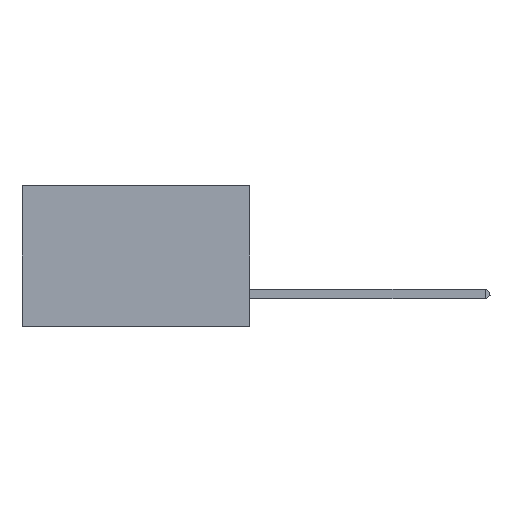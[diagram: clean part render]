
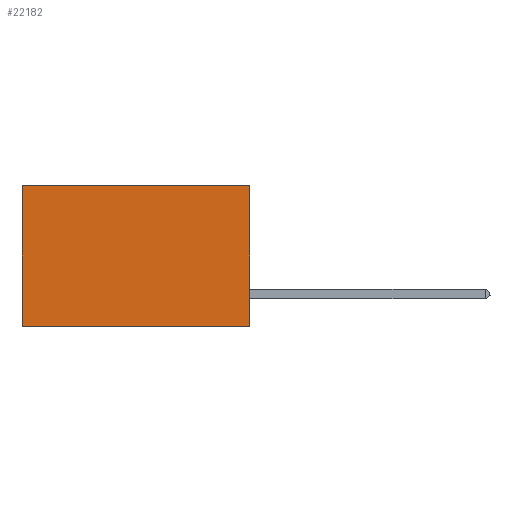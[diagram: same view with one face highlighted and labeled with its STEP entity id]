
A CAD part, left-side view. The second image highlights one B-rep face of the part: STEP entity #22182.
In plain terms, the highlighted planar face has unit normal (-1, 0, 0).
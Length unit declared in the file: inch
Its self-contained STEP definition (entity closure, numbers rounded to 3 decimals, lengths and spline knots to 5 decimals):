
#1381 = CARTESIAN_POINT ( 'NONE',  ( 0.2875, 0., 0. ) ) ;
#2530 = EDGE_CURVE ( 'NONE', #5584, #11967, #15903, .T. ) ;
#3696 = CARTESIAN_POINT ( 'NONE',  ( 0.2875, 0., 0. ) ) ;
#5584 = VERTEX_POINT ( 'NONE', #42469 ) ;
#6176 = VERTEX_POINT ( 'NONE', #1381 ) ;
#9038 = DIRECTION ( 'NONE',  ( 0., 1., 0. ) ) ;
#9777 = CARTESIAN_POINT ( 'NONE',  ( 0.2875, 0., 0. ) ) ;
#10625 = AXIS2_PLACEMENT_3D ( 'NONE', #9777, #30399, #16375 ) ;
#11967 = VERTEX_POINT ( 'NONE', #37826 ) ;
#15903 = LINE ( 'NONE', #29360, #16927 ) ;
#16375 = DIRECTION ( 'NONE',  ( 0., 0., -1. ) ) ;
#16927 = VECTOR ( 'NONE', #19357, 39.37008 ) ;
#17465 = EDGE_CURVE ( 'NONE', #6176, #38184, #38707, .T. ) ;
#18016 = CARTESIAN_POINT ( 'NONE',  ( 0.2875, 0.6, 0. ) ) ;
#19357 = DIRECTION ( 'NONE',  ( 0., 1., 0. ) ) ;
#21049 = VECTOR ( 'NONE', #37871, 39.37008 ) ;
#22182 = ADVANCED_FACE ( 'NONE', ( #33643 ), #40697, .F. ) ;
#22336 = CARTESIAN_POINT ( 'NONE',  ( 0.2875, 0., 0. ) ) ;
#25047 = ORIENTED_EDGE ( 'NONE', *, *, #17465, .T. ) ;
#25742 = VECTOR ( 'NONE', #9038, 39.37008 ) ;
#27446 = ORIENTED_EDGE ( 'NONE', *, *, #2530, .F. ) ;
#28532 = LINE ( 'NONE', #3696, #40896 ) ;
#29360 = CARTESIAN_POINT ( 'NONE',  ( 0.2875, 0., -0.37 ) ) ;
#29635 = EDGE_LOOP ( 'NONE', ( #36878, #27446, #32211, #25047 ) ) ;
#30077 = DIRECTION ( 'NONE',  ( 0., 0., -1. ) ) ;
#30399 = DIRECTION ( 'NONE',  ( 1., 0., 0. ) ) ;
#32211 = ORIENTED_EDGE ( 'NONE', *, *, #33619, .F. ) ;
#33619 = EDGE_CURVE ( 'NONE', #6176, #5584, #28532, .T. ) ;
#33643 = FACE_OUTER_BOUND ( 'NONE', #29635, .T. ) ;
#36878 = ORIENTED_EDGE ( 'NONE', *, *, #37088, .T. ) ;
#37088 = EDGE_CURVE ( 'NONE', #38184, #11967, #40721, .T. ) ;
#37343 = CARTESIAN_POINT ( 'NONE',  ( 0.2875, 0.6, 0. ) ) ;
#37826 = CARTESIAN_POINT ( 'NONE',  ( 0.2875, 0.6, -0.37 ) ) ;
#37871 = DIRECTION ( 'NONE',  ( 0., 0., -1. ) ) ;
#38184 = VERTEX_POINT ( 'NONE', #37343 ) ;
#38707 = LINE ( 'NONE', #22336, #25742 ) ;
#40697 = PLANE ( 'NONE',  #10625 ) ;
#40721 = LINE ( 'NONE', #18016, #21049 ) ;
#40896 = VECTOR ( 'NONE', #30077, 39.37008 ) ;
#42469 = CARTESIAN_POINT ( 'NONE',  ( 0.2875, 0., -0.37 ) ) ;
